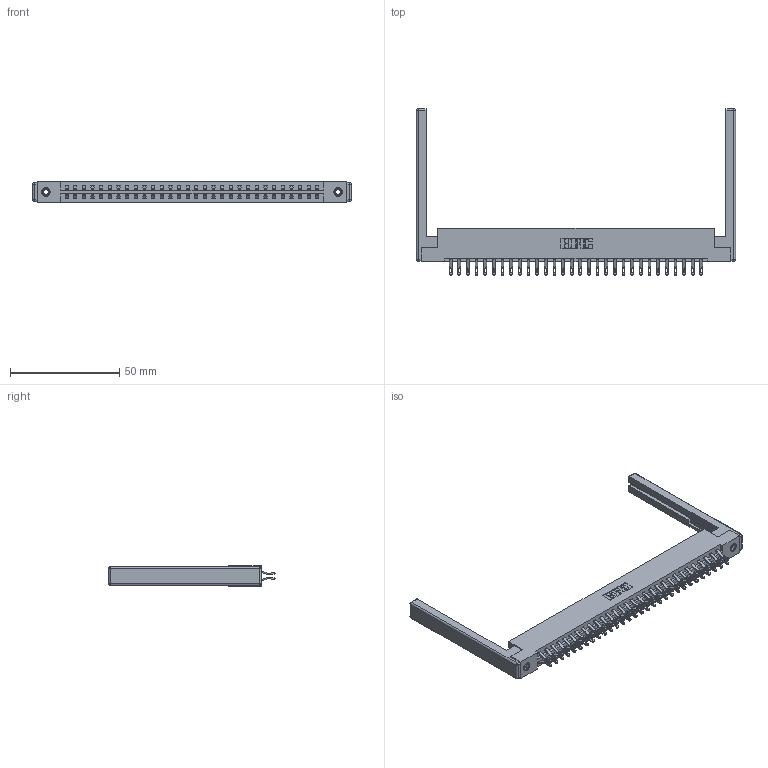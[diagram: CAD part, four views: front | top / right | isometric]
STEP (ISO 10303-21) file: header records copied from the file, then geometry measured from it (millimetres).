
FILE_DESCRIPTION (( 'STEP AP203' ), '1' );
FILE_NAME ('387-060-555-268.STEP', '2019-10-19T13:57:57', ( '' ), ( '' ), 'SwSTEP 2.0', 'SolidWorks 2016', '' );
FILE_SCHEMA (( 'CONFIG_CONTROL_DESIGN' ));
Length unit declared in the file: inch
Products named in the file (5): 345-292-001_555 Tail; 307-220-068; 337 Part_Flush Mounting Lugs - 0.156 Dia-TI; 387-060-555-268; 345-250-001_345-250-001-102
Assembly tree (65 placements, depth 2):
  387-060-555-268
    337 Part_Flush Mounting Lugs - 0.156 Dia-TI
    345-292-001_555 Tail  x60
    345-250-001_345-250-001-102  x2
    307-220-068  x2
Bounding box: 146.3 x 76.21 x 9.4 mm (x, y, z)
Volume: 19817.8 mm3; surface area: 22020.7 mm2
Topology: 65 solids, 65 shells, 3868 faces, 12041 edges, 8006 vertices
Faces by surface type: plane 2318, cylinder 1526, cone 12, sphere 8, torus 4
Entity records: 27898 total; most frequent: CARTESIAN_POINT 4709, ORIENTED_EDGE 4604, DIRECTION 4068, EDGE_CURVE 2302, VECTOR 2104, LINE 2104, VERTEX_POINT 1526, AXIS2_PLACEMENT_3D 982
